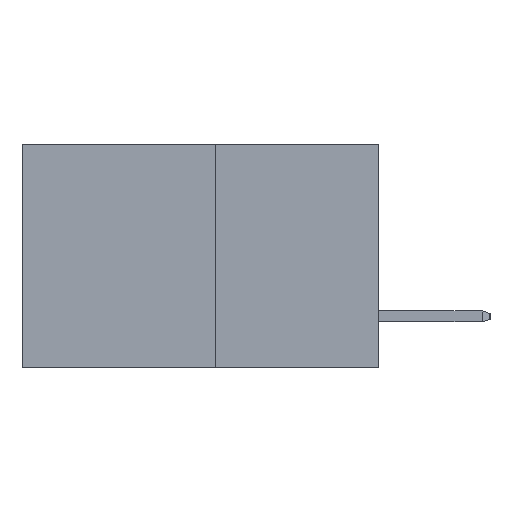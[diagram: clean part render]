
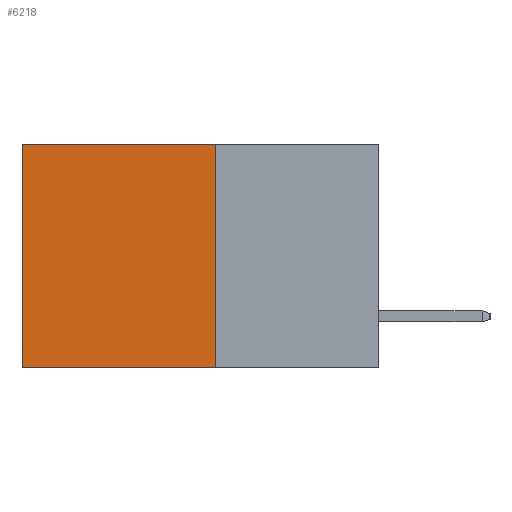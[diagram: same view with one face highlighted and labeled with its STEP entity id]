
A CAD part, left-side view. The second image highlights one B-rep face of the part: STEP entity #6218.
In plain terms, the highlighted planar face has unit normal (-1, 0, 0).
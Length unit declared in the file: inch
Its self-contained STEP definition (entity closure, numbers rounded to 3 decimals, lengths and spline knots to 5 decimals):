
#2583 = EDGE_CURVE ( 'NONE', #12933, #3455, #9760, .T. ) ;
#3337 = DIRECTION ( 'NONE',  ( 0., 1., 0. ) ) ;
#3428 = VECTOR ( 'NONE', #23753, 39.37008 ) ;
#3455 = VERTEX_POINT ( 'NONE', #5938 ) ;
#5413 = ORIENTED_EDGE ( 'NONE', *, *, #9926, .T. ) ;
#5501 = LINE ( 'NONE', #16705, #20553 ) ;
#5938 = CARTESIAN_POINT ( 'NONE',  ( 0.277, 0.27, -0.37 ) ) ;
#6218 = ADVANCED_FACE ( 'NONE', ( #20394 ), #7386, .F. ) ;
#7300 = DIRECTION ( 'NONE',  ( 0., 0., -1. ) ) ;
#7330 = DIRECTION ( 'NONE',  ( 1., 0., 0. ) ) ;
#7386 = PLANE ( 'NONE',  #14575 ) ;
#7469 = CARTESIAN_POINT ( 'NONE',  ( 0.277, 0.27, -0.37 ) ) ;
#8811 = CARTESIAN_POINT ( 'NONE',  ( 0.277, 0.27, 0. ) ) ;
#8892 = VERTEX_POINT ( 'NONE', #22986 ) ;
#9251 = LINE ( 'NONE', #8811, #3428 ) ;
#9760 = LINE ( 'NONE', #22949, #19104 ) ;
#9926 = EDGE_CURVE ( 'NONE', #12933, #8892, #9251, .T. ) ;
#10650 = DIRECTION ( 'NONE',  ( 0., 0., -1. ) ) ;
#11277 = VERTEX_POINT ( 'NONE', #18610 ) ;
#11487 = VECTOR ( 'NONE', #10650, 39.37008 ) ;
#12933 = VERTEX_POINT ( 'NONE', #19195 ) ;
#13515 = ORIENTED_EDGE ( 'NONE', *, *, #23071, .F. ) ;
#14575 = AXIS2_PLACEMENT_3D ( 'NONE', #7469, #7330, #7300 ) ;
#16445 = EDGE_CURVE ( 'NONE', #8892, #11277, #20230, .T. ) ;
#16705 = CARTESIAN_POINT ( 'NONE',  ( 0.277, 0.27, -0.37 ) ) ;
#17282 = ORIENTED_EDGE ( 'NONE', *, *, #2583, .F. ) ;
#18610 = CARTESIAN_POINT ( 'NONE',  ( 0.277, 0.59, -0.37 ) ) ;
#19104 = VECTOR ( 'NONE', #21846, 39.37008 ) ;
#19195 = CARTESIAN_POINT ( 'NONE',  ( 0.277, 0.27, 0. ) ) ;
#19953 = CARTESIAN_POINT ( 'NONE',  ( 0.277, 0.59, -0.37 ) ) ;
#20230 = LINE ( 'NONE', #19953, #11487 ) ;
#20394 = FACE_OUTER_BOUND ( 'NONE', #21162, .T. ) ;
#20553 = VECTOR ( 'NONE', #3337, 39.37008 ) ;
#20660 = ORIENTED_EDGE ( 'NONE', *, *, #16445, .T. ) ;
#21162 = EDGE_LOOP ( 'NONE', ( #20660, #13515, #17282, #5413 ) ) ;
#21846 = DIRECTION ( 'NONE',  ( 0., 0., -1. ) ) ;
#22949 = CARTESIAN_POINT ( 'NONE',  ( 0.277, 0.27, -0.37 ) ) ;
#22986 = CARTESIAN_POINT ( 'NONE',  ( 0.277, 0.59, 0. ) ) ;
#23071 = EDGE_CURVE ( 'NONE', #3455, #11277, #5501, .T. ) ;
#23753 = DIRECTION ( 'NONE',  ( 0., 1., 0. ) ) ;
